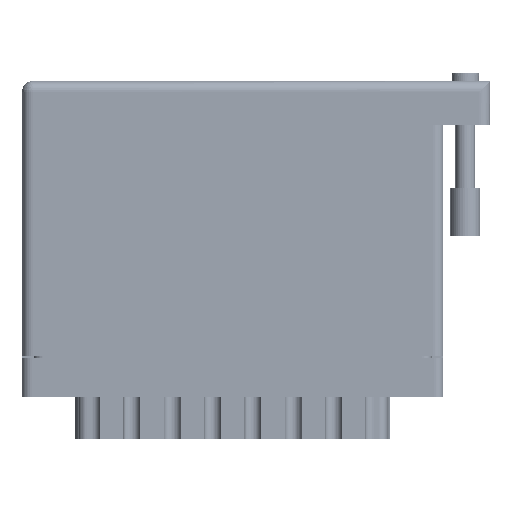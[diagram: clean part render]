
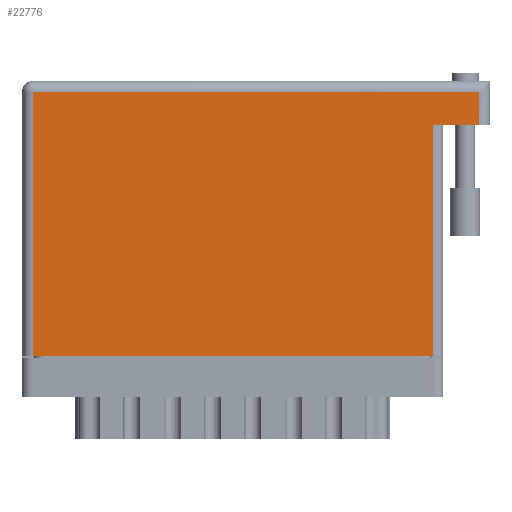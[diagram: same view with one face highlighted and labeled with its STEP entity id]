
A CAD part, front view. The second image highlights one B-rep face of the part: STEP entity #22776.
In plain terms, the highlighted face is planar.
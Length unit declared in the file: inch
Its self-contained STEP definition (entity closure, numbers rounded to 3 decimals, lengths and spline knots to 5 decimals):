
#1450 = VECTOR ( 'NONE', #22058, 39.37008 ) ;
#3459 = VERTEX_POINT ( 'NONE', #6366 ) ;
#3495 = CARTESIAN_POINT ( 'NONE',  ( 2.648, 1.495, 0. ) ) ;
#3693 = CARTESIAN_POINT ( 'NONE',  ( 0., 0., 0. ) ) ;
#4041 = VERTEX_POINT ( 'NONE', #14147 ) ;
#5675 = FACE_OUTER_BOUND ( 'NONE', #36962, .T. ) ;
#6366 = CARTESIAN_POINT ( 'NONE',  ( 2.948, 1.495, 0. ) ) ;
#8179 = DIRECTION ( 'NONE',  ( -1., 0., 0. ) ) ;
#11476 = ORIENTED_EDGE ( 'NONE', *, *, #52026, .F. ) ;
#11810 = ORIENTED_EDGE ( 'NONE', *, *, #66052, .T. ) ;
#13316 = AXIS2_PLACEMENT_3D ( 'NONE', #13476, #46692, #25016 ) ;
#13476 = CARTESIAN_POINT ( 'NONE',  ( 0., 1.775, 0. ) ) ;
#13719 = PLANE ( 'NONE',  #13316 ) ;
#14147 = CARTESIAN_POINT ( 'NONE',  ( 0.07, 0., 0. ) ) ;
#15513 = ORIENTED_EDGE ( 'NONE', *, *, #22436, .T. ) ;
#16472 = EDGE_CURVE ( 'NONE', #16959, #4041, #56942, .T. ) ;
#16959 = VERTEX_POINT ( 'NONE', #71422 ) ;
#21728 = CARTESIAN_POINT ( 'NONE',  ( 2.948, 1.705, 0. ) ) ;
#22058 = DIRECTION ( 'NONE',  ( 0., -1., 0. ) ) ;
#22436 = EDGE_CURVE ( 'NONE', #4041, #41299, #52454, .T. ) ;
#22701 = DIRECTION ( 'NONE',  ( -1., 0., 0. ) ) ;
#22776 = ADVANCED_FACE ( 'NONE', ( #5675 ), #13719, .F. ) ;
#24673 = VECTOR ( 'NONE', #53970, 39.37008 ) ;
#24950 = EDGE_CURVE ( 'NONE', #41299, #67118, #54630, .T. ) ;
#25016 = DIRECTION ( 'NONE',  ( -1., 0., 0. ) ) ;
#26283 = CARTESIAN_POINT ( 'NONE',  ( 0.07, 0., 0. ) ) ;
#26668 = CARTESIAN_POINT ( 'NONE',  ( 2.948, 1.775, 0. ) ) ;
#27879 = CARTESIAN_POINT ( 'NONE',  ( 3.018, 1.495, 0. ) ) ;
#36248 = CARTESIAN_POINT ( 'NONE',  ( 0., 1.705, 0. ) ) ;
#36461 = LINE ( 'NONE', #26668, #64605 ) ;
#36631 = CARTESIAN_POINT ( 'NONE',  ( 2.648, 1.495, 0. ) ) ;
#36962 = EDGE_LOOP ( 'NONE', ( #15513, #70373, #11476, #11810, #56923, #41194 ) ) ;
#38840 = LINE ( 'NONE', #27879, #66105 ) ;
#41194 = ORIENTED_EDGE ( 'NONE', *, *, #16472, .T. ) ;
#41299 = VERTEX_POINT ( 'NONE', #43832 ) ;
#41856 = VECTOR ( 'NONE', #56058, 39.37008 ) ;
#43832 = CARTESIAN_POINT ( 'NONE',  ( 2.648, 0., 0. ) ) ;
#44932 = EDGE_CURVE ( 'NONE', #62155, #16959, #72346, .T. ) ;
#46692 = DIRECTION ( 'NONE',  ( 0., 0., -1. ) ) ;
#52026 = EDGE_CURVE ( 'NONE', #3459, #67118, #38840, .T. ) ;
#52454 = LINE ( 'NONE', #3693, #41856 ) ;
#53970 = DIRECTION ( 'NONE',  ( 0., 1., 0. ) ) ;
#54630 = LINE ( 'NONE', #3495, #24673 ) ;
#56058 = DIRECTION ( 'NONE',  ( 1., 0., 0. ) ) ;
#56923 = ORIENTED_EDGE ( 'NONE', *, *, #44932, .T. ) ;
#56942 = LINE ( 'NONE', #26283, #1450 ) ;
#57430 = VECTOR ( 'NONE', #8179, 39.37008 ) ;
#62155 = VERTEX_POINT ( 'NONE', #21728 ) ;
#64605 = VECTOR ( 'NONE', #71158, 39.37008 ) ;
#66052 = EDGE_CURVE ( 'NONE', #3459, #62155, #36461, .T. ) ;
#66105 = VECTOR ( 'NONE', #22701, 39.37008 ) ;
#67118 = VERTEX_POINT ( 'NONE', #36631 ) ;
#70373 = ORIENTED_EDGE ( 'NONE', *, *, #24950, .T. ) ;
#71158 = DIRECTION ( 'NONE',  ( 0., 1., 0. ) ) ;
#71422 = CARTESIAN_POINT ( 'NONE',  ( 0.07, 1.705, 0. ) ) ;
#72346 = LINE ( 'NONE', #36248, #57430 ) ;
